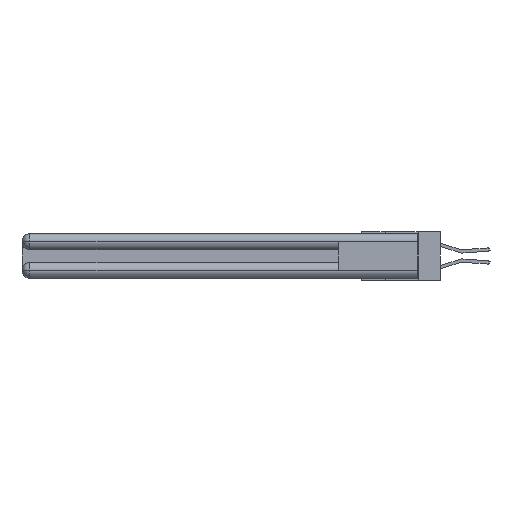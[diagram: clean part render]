
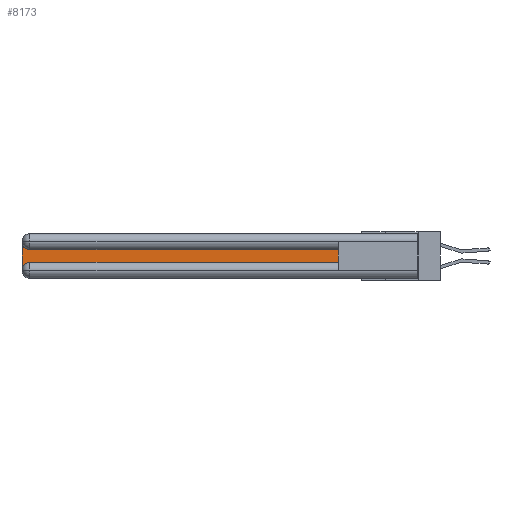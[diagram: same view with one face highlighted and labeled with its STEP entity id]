
A CAD part, left-side view. The second image highlights one B-rep face of the part: STEP entity #8173.
In plain terms, the highlighted planar face has unit normal (-1, 0, 0).
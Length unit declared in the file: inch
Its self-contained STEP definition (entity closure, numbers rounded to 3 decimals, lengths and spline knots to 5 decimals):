
#404 = ORIENTED_EDGE ( 'NONE', *, *, #22468, .T. ) ;
#1096 = CARTESIAN_POINT ( 'NONE',  ( 0.075, 0.6, -0.2175 ) ) ;
#1350 = FACE_OUTER_BOUND ( 'NONE', #9170, .T. ) ;
#2097 = CARTESIAN_POINT ( 'NONE',  ( 0.075, 3., -0.1225 ) ) ;
#2252 = AXIS2_PLACEMENT_3D ( 'NONE', #10127, #17275, #5385 ) ;
#3868 = EDGE_CURVE ( 'NONE', #21114, #6484, #10627, .T. ) ;
#4829 = VECTOR ( 'NONE', #10415, 39.37008 ) ;
#4861 = CIRCLE ( 'NONE', #21245, 0.06 ) ;
#5385 = DIRECTION ( 'NONE',  ( 0., 0., -1. ) ) ;
#5797 = CARTESIAN_POINT ( 'NONE',  ( 0.075, 0.6, -0.2175 ) ) ;
#6484 = VERTEX_POINT ( 'NONE', #29514 ) ;
#6974 = VECTOR ( 'NONE', #7841, 39.37008 ) ;
#6989 = ORIENTED_EDGE ( 'NONE', *, *, #24498, .T. ) ;
#7239 = DIRECTION ( 'NONE',  ( 0., 0., 1. ) ) ;
#7682 = LINE ( 'NONE', #1096, #19723 ) ;
#7685 = DIRECTION ( 'NONE',  ( 0., 0., -1. ) ) ;
#7841 = DIRECTION ( 'NONE',  ( 0., -1., 0. ) ) ;
#8173 = ADVANCED_FACE ( 'NONE', ( #1350 ), #30095, .F. ) ;
#8207 = VERTEX_POINT ( 'NONE', #18914 ) ;
#8784 = LINE ( 'NONE', #24168, #9143 ) ;
#9143 = VECTOR ( 'NONE', #24581, 39.37008 ) ;
#9170 = EDGE_LOOP ( 'NONE', ( #14161, #6989, #28135, #404, #17977, #25873 ) ) ;
#10127 = CARTESIAN_POINT ( 'NONE',  ( 0.075, 2.94, -0.2775 ) ) ;
#10415 = DIRECTION ( 'NONE',  ( 0., 1., 0. ) ) ;
#10627 = LINE ( 'NONE', #23234, #4829 ) ;
#11506 = EDGE_CURVE ( 'NONE', #12763, #23958, #8784, .T. ) ;
#12522 = EDGE_CURVE ( 'NONE', #8207, #22892, #16794, .T. ) ;
#12713 = CARTESIAN_POINT ( 'NONE',  ( 0.075, 0.6, -0.2175 ) ) ;
#12763 = VERTEX_POINT ( 'NONE', #25568 ) ;
#14161 = ORIENTED_EDGE ( 'NONE', *, *, #3868, .T. ) ;
#14917 = CARTESIAN_POINT ( 'NONE',  ( 0.075, 2.94, -0.0625 ) ) ;
#16794 = LINE ( 'NONE', #12713, #6974 ) ;
#17275 = DIRECTION ( 'NONE',  ( 1., 0., 0. ) ) ;
#17956 = CARTESIAN_POINT ( 'NONE',  ( 0.075, 0.6, -0.1225 ) ) ;
#17977 = ORIENTED_EDGE ( 'NONE', *, *, #12522, .T. ) ;
#18012 = EDGE_CURVE ( 'NONE', #22892, #21114, #7682, .T. ) ;
#18914 = CARTESIAN_POINT ( 'NONE',  ( 0.075, 2.94, -0.2175 ) ) ;
#19723 = VECTOR ( 'NONE', #7239, 39.37008 ) ;
#20753 = DIRECTION ( 'NONE',  ( 1., 0., 0. ) ) ;
#21114 = VERTEX_POINT ( 'NONE', #17956 ) ;
#21245 = AXIS2_PLACEMENT_3D ( 'NONE', #14917, #21847, #7685 ) ;
#21847 = DIRECTION ( 'NONE',  ( 1., 0., 0. ) ) ;
#22468 = EDGE_CURVE ( 'NONE', #23958, #8207, #26528, .T. ) ;
#22892 = VERTEX_POINT ( 'NONE', #5797 ) ;
#23110 = DIRECTION ( 'NONE',  ( 0., 0., -1. ) ) ;
#23234 = CARTESIAN_POINT ( 'NONE',  ( 0.075, 0.6, -0.1225 ) ) ;
#23958 = VERTEX_POINT ( 'NONE', #26224 ) ;
#24168 = CARTESIAN_POINT ( 'NONE',  ( 0.075, 3., -0.2175 ) ) ;
#24498 = EDGE_CURVE ( 'NONE', #6484, #12763, #4861, .T. ) ;
#24523 = AXIS2_PLACEMENT_3D ( 'NONE', #2097, #20753, #23110 ) ;
#24581 = DIRECTION ( 'NONE',  ( 0., 0., -1. ) ) ;
#25568 = CARTESIAN_POINT ( 'NONE',  ( 0.075, 3., -0.0625 ) ) ;
#25873 = ORIENTED_EDGE ( 'NONE', *, *, #18012, .T. ) ;
#26224 = CARTESIAN_POINT ( 'NONE',  ( 0.075, 3., -0.2775 ) ) ;
#26528 = CIRCLE ( 'NONE', #2252, 0.06 ) ;
#28135 = ORIENTED_EDGE ( 'NONE', *, *, #11506, .T. ) ;
#29514 = CARTESIAN_POINT ( 'NONE',  ( 0.075, 2.94, -0.1225 ) ) ;
#30095 = PLANE ( 'NONE',  #24523 ) ;
